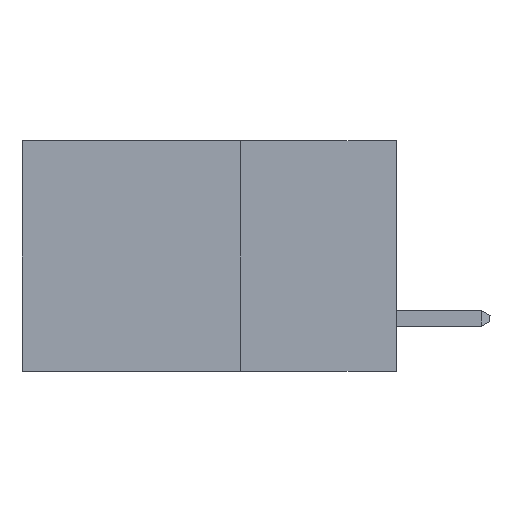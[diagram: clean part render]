
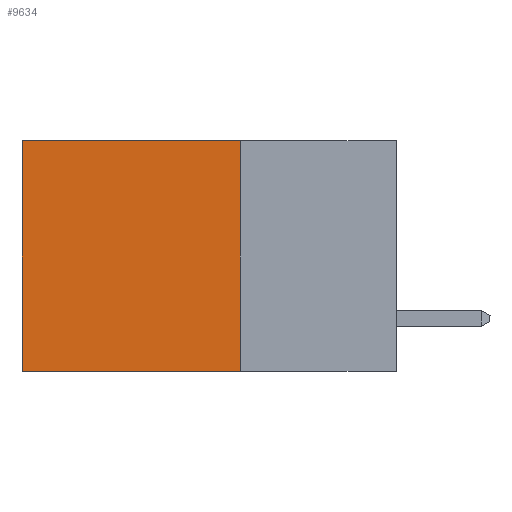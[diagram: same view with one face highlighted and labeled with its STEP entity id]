
A CAD part, left-side view. The second image highlights one B-rep face of the part: STEP entity #9634.
In plain terms, the highlighted planar face has unit normal (-1, 0, 0).
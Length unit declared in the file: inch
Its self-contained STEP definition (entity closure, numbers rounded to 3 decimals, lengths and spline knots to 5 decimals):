
#639 = FACE_OUTER_BOUND ( 'NONE', #9743, .T. ) ;
#1091 = CARTESIAN_POINT ( 'NONE',  ( 0.2615, 0.25, 0. ) ) ;
#1538 = PLANE ( 'NONE',  #5668 ) ;
#1579 = VECTOR ( 'NONE', #15989, 39.37008 ) ;
#1901 = DIRECTION ( 'NONE',  ( 0., 1., 0. ) ) ;
#2376 = CARTESIAN_POINT ( 'NONE',  ( 0.2615, 0.25, -0.37 ) ) ;
#2427 = VECTOR ( 'NONE', #17897, 39.37008 ) ;
#3180 = DIRECTION ( 'NONE',  ( 1., 0., 0. ) ) ;
#4319 = CARTESIAN_POINT ( 'NONE',  ( 0.2615, 0.6, 0. ) ) ;
#5229 = VERTEX_POINT ( 'NONE', #2376 ) ;
#5668 = AXIS2_PLACEMENT_3D ( 'NONE', #6177, #3180, #14621 ) ;
#6177 = CARTESIAN_POINT ( 'NONE',  ( 0.2615, 0.25, -0.37 ) ) ;
#6664 = CARTESIAN_POINT ( 'NONE',  ( 0.2615, 0.25, -0.37 ) ) ;
#7680 = EDGE_CURVE ( 'NONE', #12979, #18453, #14109, .T. ) ;
#9570 = ORIENTED_EDGE ( 'NONE', *, *, #19957, .F. ) ;
#9634 = ADVANCED_FACE ( 'NONE', ( #639 ), #1538, .F. ) ;
#9647 = VECTOR ( 'NONE', #13109, 39.37008 ) ;
#9743 = EDGE_LOOP ( 'NONE', ( #10109, #9570, #19565, #11526 ) ) ;
#10109 = ORIENTED_EDGE ( 'NONE', *, *, #7680, .T. ) ;
#11050 = CARTESIAN_POINT ( 'NONE',  ( 0.2615, 0.25, 0. ) ) ;
#11526 = ORIENTED_EDGE ( 'NONE', *, *, #17359, .T. ) ;
#12979 = VERTEX_POINT ( 'NONE', #4319 ) ;
#13109 = DIRECTION ( 'NONE',  ( 0., 0., -1. ) ) ;
#14109 = LINE ( 'NONE', #19538, #9647 ) ;
#14621 = DIRECTION ( 'NONE',  ( 0., 0., -1. ) ) ;
#15441 = LINE ( 'NONE', #16269, #2427 ) ;
#15794 = EDGE_CURVE ( 'NONE', #19647, #5229, #15441, .T. ) ;
#15856 = CARTESIAN_POINT ( 'NONE',  ( 0.2615, 0.6, -0.37 ) ) ;
#15989 = DIRECTION ( 'NONE',  ( 0., 1., 0. ) ) ;
#16159 = VECTOR ( 'NONE', #1901, 39.37008 ) ;
#16269 = CARTESIAN_POINT ( 'NONE',  ( 0.2615, 0.25, -0.37 ) ) ;
#17359 = EDGE_CURVE ( 'NONE', #19647, #12979, #18909, .T. ) ;
#17897 = DIRECTION ( 'NONE',  ( 0., 0., -1. ) ) ;
#18453 = VERTEX_POINT ( 'NONE', #15856 ) ;
#18909 = LINE ( 'NONE', #11050, #1579 ) ;
#19538 = CARTESIAN_POINT ( 'NONE',  ( 0.2615, 0.6, -0.37 ) ) ;
#19565 = ORIENTED_EDGE ( 'NONE', *, *, #15794, .F. ) ;
#19647 = VERTEX_POINT ( 'NONE', #1091 ) ;
#19957 = EDGE_CURVE ( 'NONE', #5229, #18453, #20376, .T. ) ;
#20376 = LINE ( 'NONE', #6664, #16159 ) ;
